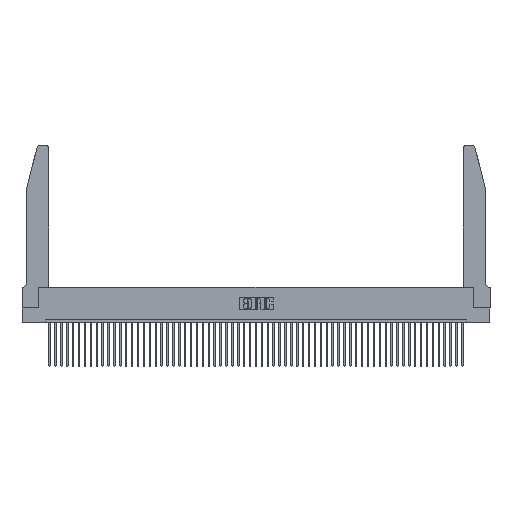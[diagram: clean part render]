
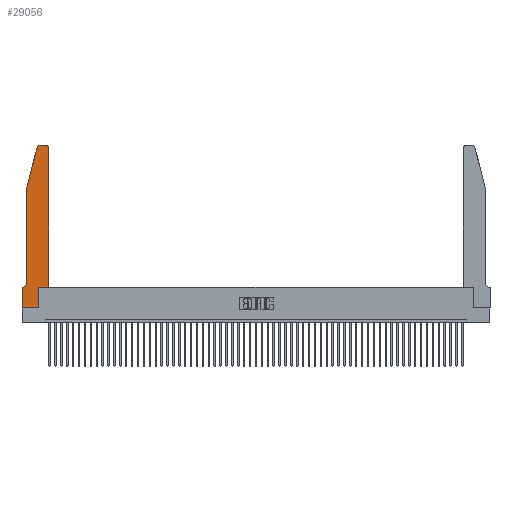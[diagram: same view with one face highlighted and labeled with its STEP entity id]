
A CAD part, top view. The second image highlights one B-rep face of the part: STEP entity #29056.
In plain terms, the highlighted planar face has unit normal (0, 0, 1).
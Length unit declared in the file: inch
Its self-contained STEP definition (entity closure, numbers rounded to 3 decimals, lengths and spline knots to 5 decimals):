
#570 = VERTEX_POINT ( 'NONE', #25438 ) ;
#1098 = CARTESIAN_POINT ( 'NONE',  ( 0.0755, 0.42, 0.37 ) ) ;
#1231 = VERTEX_POINT ( 'NONE', #29436 ) ;
#1372 = ORIENTED_EDGE ( 'NONE', *, *, #22085, .T. ) ;
#1415 = CARTESIAN_POINT ( 'NONE',  ( 0.0755, 2., 0.37 ) ) ;
#1733 = DIRECTION ( 'NONE',  ( 1., 0., 0. ) ) ;
#1750 = AXIS2_PLACEMENT_3D ( 'NONE', #30017, #8951, #8616 ) ;
#1811 = ORIENTED_EDGE ( 'NONE', *, *, #9735, .T. ) ;
#2393 = CARTESIAN_POINT ( 'NONE',  ( 0.4505, 0.35, 0.37 ) ) ;
#2950 = ORIENTED_EDGE ( 'NONE', *, *, #49884, .T. ) ;
#3002 = VERTEX_POINT ( 'NONE', #41538 ) ;
#3852 = CARTESIAN_POINT ( 'NONE',  ( 0.284, 2.75, 0.37 ) ) ;
#3882 = EDGE_CURVE ( 'NONE', #23890, #5228, #34756, .T. ) ;
#4083 = ORIENTED_EDGE ( 'NONE', *, *, #44065, .T. ) ;
#4596 = VECTOR ( 'NONE', #26031, 39.37008 ) ;
#5201 = ORIENTED_EDGE ( 'NONE', *, *, #15659, .T. ) ;
#5228 = VERTEX_POINT ( 'NONE', #31514 ) ;
#5718 = DIRECTION ( 'NONE',  ( -0.239, -0.971, 0. ) ) ;
#7991 = VECTOR ( 'NONE', #14277, 39.37008 ) ;
#8012 = VERTEX_POINT ( 'NONE', #52107 ) ;
#8119 = DIRECTION ( 'NONE',  ( 1., 0., 0. ) ) ;
#8122 = VECTOR ( 'NONE', #5718, 39.37008 ) ;
#8130 = CARTESIAN_POINT ( 'NONE',  ( 0.4505, 0.35, 0.37 ) ) ;
#8616 = DIRECTION ( 'NONE',  ( 1., 0., 0. ) ) ;
#8951 = DIRECTION ( 'NONE',  ( 0., 0., 1. ) ) ;
#9135 = VECTOR ( 'NONE', #16215, 39.37008 ) ;
#9400 = ORIENTED_EDGE ( 'NONE', *, *, #32325, .T. ) ;
#9735 = EDGE_CURVE ( 'NONE', #18539, #3002, #16461, .T. ) ;
#10798 = LINE ( 'NONE', #53150, #19303 ) ;
#11525 = DIRECTION ( 'NONE',  ( 0., -1., 0. ) ) ;
#12190 = CARTESIAN_POINT ( 'NONE',  ( 0.0755, 0.35, 0.37 ) ) ;
#14242 = CARTESIAN_POINT ( 'NONE',  ( 0.0055, 0.42, 0.37 ) ) ;
#14256 = CARTESIAN_POINT ( 'NONE',  ( 0.2865, 0., 0.37 ) ) ;
#14277 = DIRECTION ( 'NONE',  ( 0., 1., 0. ) ) ;
#15659 = EDGE_CURVE ( 'NONE', #51980, #33629, #38147, .T. ) ;
#16215 = DIRECTION ( 'NONE',  ( -1., 0., 0. ) ) ;
#16312 = ORIENTED_EDGE ( 'NONE', *, *, #16408, .T. ) ;
#16408 = EDGE_CURVE ( 'NONE', #570, #51980, #17015, .T. ) ;
#16461 = LINE ( 'NONE', #12190, #9135 ) ;
#16875 = DIRECTION ( 'NONE',  ( 0., 0., 1. ) ) ;
#17015 = LINE ( 'NONE', #22051, #27554 ) ;
#18331 = CARTESIAN_POINT ( 'NONE',  ( 0.2865, 0.35, 0.37 ) ) ;
#18386 = VERTEX_POINT ( 'NONE', #3852 ) ;
#18539 = VERTEX_POINT ( 'NONE', #52343 ) ;
#18819 = DIRECTION ( 'NONE',  ( 1., 0., 0. ) ) ;
#19303 = VECTOR ( 'NONE', #11525, 39.37008 ) ;
#21629 = CARTESIAN_POINT ( 'NONE',  ( 0.0755, 2., 0.37 ) ) ;
#21816 = FACE_OUTER_BOUND ( 'NONE', #34365, .T. ) ;
#22051 = CARTESIAN_POINT ( 'NONE',  ( 0., 0., 0.37 ) ) ;
#22085 = EDGE_CURVE ( 'NONE', #33629, #23890, #43098, .T. ) ;
#22492 = CARTESIAN_POINT ( 'NONE',  ( 0.2865, 0.35, 0.37 ) ) ;
#22788 = ORIENTED_EDGE ( 'NONE', *, *, #24991, .T. ) ;
#23022 = EDGE_CURVE ( 'NONE', #18386, #8012, #25976, .T. ) ;
#23890 = VERTEX_POINT ( 'NONE', #8130 ) ;
#24176 = PLANE ( 'NONE',  #42221 ) ;
#24564 = CARTESIAN_POINT ( 'NONE',  ( 0., 0.35, 0.37 ) ) ;
#24991 = EDGE_CURVE ( 'NONE', #3002, #570, #10798, .T. ) ;
#25348 = CIRCLE ( 'NONE', #1750, 0.03 ) ;
#25438 = CARTESIAN_POINT ( 'NONE',  ( 0., 0., 0.37 ) ) ;
#25976 = CIRCLE ( 'NONE', #31899, 0.03 ) ;
#26031 = DIRECTION ( 'NONE',  ( 0., -1., 0. ) ) ;
#27554 = VECTOR ( 'NONE', #1733, 39.37008 ) ;
#29056 = ADVANCED_FACE ( 'NONE', ( #21816 ), #24176, .T. ) ;
#29173 = DIRECTION ( 'NONE',  ( 0., 0., 1. ) ) ;
#29436 = CARTESIAN_POINT ( 'NONE',  ( 0.0755, 2., 0.37 ) ) ;
#29982 = EDGE_CURVE ( 'NONE', #8012, #1231, #30307, .T. ) ;
#30017 = CARTESIAN_POINT ( 'NONE',  ( 0.4205, 2.72, 0.37 ) ) ;
#30307 = LINE ( 'NONE', #1415, #8122 ) ;
#30390 = AXIS2_PLACEMENT_3D ( 'NONE', #14242, #52004, #35191 ) ;
#31341 = EDGE_CURVE ( 'NONE', #34774, #18386, #34733, .T. ) ;
#31514 = CARTESIAN_POINT ( 'NONE',  ( 0.4505, 2.72, 0.37 ) ) ;
#31899 = AXIS2_PLACEMENT_3D ( 'NONE', #44572, #16875, #34785 ) ;
#32325 = EDGE_CURVE ( 'NONE', #53951, #18539, #51086, .T. ) ;
#33551 = ORIENTED_EDGE ( 'NONE', *, *, #31341, .T. ) ;
#33629 = VERTEX_POINT ( 'NONE', #22492 ) ;
#33835 = ORIENTED_EDGE ( 'NONE', *, *, #29982, .T. ) ;
#34237 = CARTESIAN_POINT ( 'NONE',  ( 0.4205, 2.75, 0.37 ) ) ;
#34365 = EDGE_LOOP ( 'NONE', ( #33551, #41451, #33835, #4083, #9400, #1811, #22788, #16312, #5201, #1372, #40920, #2950 ) ) ;
#34733 = LINE ( 'NONE', #42367, #53899 ) ;
#34756 = LINE ( 'NONE', #47466, #7991 ) ;
#34774 = VERTEX_POINT ( 'NONE', #34237 ) ;
#34785 = DIRECTION ( 'NONE',  ( 1., 0., 0. ) ) ;
#35191 = DIRECTION ( 'NONE',  ( -1., 0., 0. ) ) ;
#35467 = DIRECTION ( 'NONE',  ( 0., 1., 0. ) ) ;
#38072 = LINE ( 'NONE', #21629, #4596 ) ;
#38147 = LINE ( 'NONE', #18331, #51095 ) ;
#40920 = ORIENTED_EDGE ( 'NONE', *, *, #3882, .T. ) ;
#41451 = ORIENTED_EDGE ( 'NONE', *, *, #23022, .T. ) ;
#41538 = CARTESIAN_POINT ( 'NONE',  ( 0., 0.35, 0.37 ) ) ;
#42221 = AXIS2_PLACEMENT_3D ( 'NONE', #24564, #29173, #8119 ) ;
#42367 = CARTESIAN_POINT ( 'NONE',  ( 0.2605, 2.75, 0.37 ) ) ;
#43098 = LINE ( 'NONE', #2393, #53080 ) ;
#44065 = EDGE_CURVE ( 'NONE', #1231, #53951, #38072, .T. ) ;
#44572 = CARTESIAN_POINT ( 'NONE',  ( 0.284, 2.72, 0.37 ) ) ;
#47466 = CARTESIAN_POINT ( 'NONE',  ( 0.4505, 0.35, 0.37 ) ) ;
#49884 = EDGE_CURVE ( 'NONE', #5228, #34774, #25348, .T. ) ;
#50327 = DIRECTION ( 'NONE',  ( -1., 0., 0. ) ) ;
#51086 = CIRCLE ( 'NONE', #30390, 0.07 ) ;
#51095 = VECTOR ( 'NONE', #35467, 39.37008 ) ;
#51980 = VERTEX_POINT ( 'NONE', #14256 ) ;
#52004 = DIRECTION ( 'NONE',  ( 0., 0., -1. ) ) ;
#52107 = CARTESIAN_POINT ( 'NONE',  ( 0.25487, 2.72718, 0.37 ) ) ;
#52343 = CARTESIAN_POINT ( 'NONE',  ( 0.0055, 0.35, 0.37 ) ) ;
#53080 = VECTOR ( 'NONE', #18819, 39.37008 ) ;
#53150 = CARTESIAN_POINT ( 'NONE',  ( 0., 0., 0.37 ) ) ;
#53899 = VECTOR ( 'NONE', #50327, 39.37008 ) ;
#53951 = VERTEX_POINT ( 'NONE', #1098 ) ;
